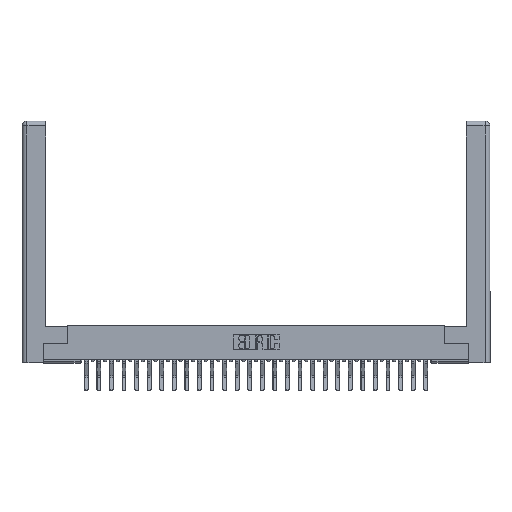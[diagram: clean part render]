
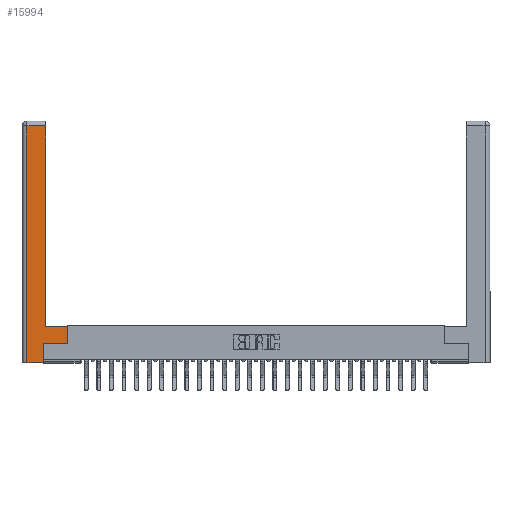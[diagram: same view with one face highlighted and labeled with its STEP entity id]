
A CAD part, top view. The second image highlights one B-rep face of the part: STEP entity #15994.
In plain terms, the highlighted planar face has unit normal (0, 0, 1).
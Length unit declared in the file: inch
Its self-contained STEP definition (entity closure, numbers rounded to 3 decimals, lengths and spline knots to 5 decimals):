
#858 = CARTESIAN_POINT ( 'NONE',  ( 0.295, 0.45, 0. ) ) ;
#1131 = ORIENTED_EDGE ( 'NONE', *, *, #8397, .T. ) ;
#1596 = EDGE_LOOP ( 'NONE', ( #13657, #1131, #10730, #4633, #23025, #2570, #13621, #4463 ) ) ;
#1673 = LINE ( 'NONE', #858, #28961 ) ;
#1866 = EDGE_CURVE ( 'NONE', #18618, #10944, #4181, .T. ) ;
#1971 = EDGE_CURVE ( 'NONE', #16555, #18618, #26498, .T. ) ;
#2566 = LINE ( 'NONE', #21732, #20310 ) ;
#2570 = ORIENTED_EDGE ( 'NONE', *, *, #1866, .T. ) ;
#2589 = CARTESIAN_POINT ( 'NONE',  ( 0.0615, 0., 0. ) ) ;
#2773 = DIRECTION ( 'NONE',  ( 1., 0., 0. ) ) ;
#2801 = PLANE ( 'NONE',  #21403 ) ;
#2844 = CARTESIAN_POINT ( 'NONE',  ( 0.295, 3., 0. ) ) ;
#3001 = EDGE_CURVE ( 'NONE', #6743, #5440, #4983, .T. ) ;
#4181 = LINE ( 'NONE', #7737, #9872 ) ;
#4325 = VECTOR ( 'NONE', #2773, 39.37008 ) ;
#4463 = ORIENTED_EDGE ( 'NONE', *, *, #12105, .T. ) ;
#4633 = ORIENTED_EDGE ( 'NONE', *, *, #8508, .T. ) ;
#4983 = LINE ( 'NONE', #2589, #21660 ) ;
#5440 = VERTEX_POINT ( 'NONE', #12868 ) ;
#5494 = DIRECTION ( 'NONE',  ( -1., 0., 0. ) ) ;
#5991 = DIRECTION ( 'NONE',  ( 0., 1., 0. ) ) ;
#6562 = FACE_OUTER_BOUND ( 'NONE', #1596, .T. ) ;
#6729 = LINE ( 'NONE', #21755, #24800 ) ;
#6743 = VERTEX_POINT ( 'NONE', #21914 ) ;
#7649 = CARTESIAN_POINT ( 'NONE',  ( 0.265, 0., 0. ) ) ;
#7737 = CARTESIAN_POINT ( 'NONE',  ( 0.565, 0.245, 0. ) ) ;
#8032 = DIRECTION ( 'NONE',  ( 0., 1., 0. ) ) ;
#8106 = VECTOR ( 'NONE', #8032, 39.37008 ) ;
#8397 = EDGE_CURVE ( 'NONE', #18725, #6743, #2566, .T. ) ;
#8508 = EDGE_CURVE ( 'NONE', #5440, #16555, #16030, .T. ) ;
#9872 = VECTOR ( 'NONE', #23567, 39.37008 ) ;
#10086 = DIRECTION ( 'NONE',  ( 0., 1., 0. ) ) ;
#10730 = ORIENTED_EDGE ( 'NONE', *, *, #3001, .T. ) ;
#10932 = EDGE_CURVE ( 'NONE', #28137, #18725, #22988, .T. ) ;
#10944 = VERTEX_POINT ( 'NONE', #27931 ) ;
#12105 = EDGE_CURVE ( 'NONE', #27151, #28137, #1673, .T. ) ;
#12169 = DIRECTION ( 'NONE',  ( -1., 0., 0. ) ) ;
#12868 = CARTESIAN_POINT ( 'NONE',  ( 0.0615, 0., 0. ) ) ;
#13290 = CARTESIAN_POINT ( 'NONE',  ( 0.295, 0.45, 0. ) ) ;
#13621 = ORIENTED_EDGE ( 'NONE', *, *, #17562, .T. ) ;
#13657 = ORIENTED_EDGE ( 'NONE', *, *, #10932, .T. ) ;
#15585 = CARTESIAN_POINT ( 'NONE',  ( 0.295, 2.94, 0. ) ) ;
#15994 = ADVANCED_FACE ( 'NONE', ( #6562 ), #2801, .F. ) ;
#16030 = LINE ( 'NONE', #22980, #4325 ) ;
#16555 = VERTEX_POINT ( 'NONE', #7649 ) ;
#17562 = EDGE_CURVE ( 'NONE', #10944, #27151, #6729, .T. ) ;
#18464 = DIRECTION ( 'NONE',  ( 0., -1., 0. ) ) ;
#18618 = VERTEX_POINT ( 'NONE', #26282 ) ;
#18725 = VERTEX_POINT ( 'NONE', #15585 ) ;
#19355 = DIRECTION ( 'NONE',  ( -1., 0., 0. ) ) ;
#20310 = VECTOR ( 'NONE', #19355, 39.37008 ) ;
#21192 = CARTESIAN_POINT ( 'NONE',  ( 0.565, 0.45, 0. ) ) ;
#21403 = AXIS2_PLACEMENT_3D ( 'NONE', #23303, #27792, #5494 ) ;
#21598 = CARTESIAN_POINT ( 'NONE',  ( 0.265, 0.245, 0. ) ) ;
#21660 = VECTOR ( 'NONE', #18464, 39.37008 ) ;
#21732 = CARTESIAN_POINT ( 'NONE',  ( 0.0615, 2.94, 0. ) ) ;
#21755 = CARTESIAN_POINT ( 'NONE',  ( 0.565, 0.45, 0. ) ) ;
#21914 = CARTESIAN_POINT ( 'NONE',  ( 0.0615, 2.94, 0. ) ) ;
#22980 = CARTESIAN_POINT ( 'NONE',  ( 0.265, 0., 0. ) ) ;
#22988 = LINE ( 'NONE', #2844, #29384 ) ;
#23025 = ORIENTED_EDGE ( 'NONE', *, *, #1971, .T. ) ;
#23303 = CARTESIAN_POINT ( 'NONE',  ( 0., 0., 0. ) ) ;
#23567 = DIRECTION ( 'NONE',  ( 1., 0., 0. ) ) ;
#24800 = VECTOR ( 'NONE', #5991, 39.37008 ) ;
#26282 = CARTESIAN_POINT ( 'NONE',  ( 0.265, 0.245, 0. ) ) ;
#26498 = LINE ( 'NONE', #21598, #8106 ) ;
#27151 = VERTEX_POINT ( 'NONE', #21192 ) ;
#27792 = DIRECTION ( 'NONE',  ( 0., 0., -1. ) ) ;
#27931 = CARTESIAN_POINT ( 'NONE',  ( 0.565, 0.245, 0. ) ) ;
#28137 = VERTEX_POINT ( 'NONE', #13290 ) ;
#28961 = VECTOR ( 'NONE', #12169, 39.37008 ) ;
#29384 = VECTOR ( 'NONE', #10086, 39.37008 ) ;
